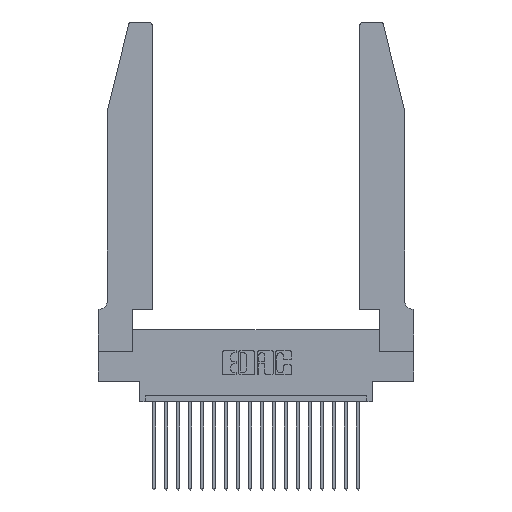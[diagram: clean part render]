
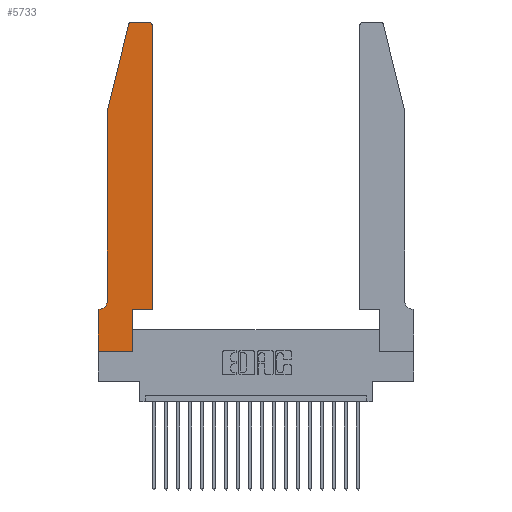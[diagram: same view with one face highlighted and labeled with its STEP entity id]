
A CAD part, top view. The second image highlights one B-rep face of the part: STEP entity #5733.
In plain terms, the highlighted planar face has unit normal (0, 0, 1).
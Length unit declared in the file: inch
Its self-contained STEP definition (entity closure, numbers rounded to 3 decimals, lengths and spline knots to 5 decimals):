
#172 = EDGE_CURVE ( 'NONE', #2098, #2395, #539, .T. ) ;
#305 = LINE ( 'NONE', #10975, #13659 ) ;
#336 = DIRECTION ( 'NONE',  ( -1., 0., 0. ) ) ;
#539 = LINE ( 'NONE', #12052, #19403 ) ;
#838 = LINE ( 'NONE', #2893, #16295 ) ;
#889 = EDGE_CURVE ( 'NONE', #14519, #3531, #14907, .T. ) ;
#1054 = EDGE_CURVE ( 'NONE', #8206, #13975, #4939, .T. ) ;
#1681 = ORIENTED_EDGE ( 'NONE', *, *, #889, .T. ) ;
#2098 = VERTEX_POINT ( 'NONE', #4313 ) ;
#2245 = ORIENTED_EDGE ( 'NONE', *, *, #15053, .T. ) ;
#2393 = AXIS2_PLACEMENT_3D ( 'NONE', #4122, #5932, #5784 ) ;
#2395 = VERTEX_POINT ( 'NONE', #18544 ) ;
#2477 = LINE ( 'NONE', #9210, #20814 ) ;
#2893 = CARTESIAN_POINT ( 'NONE',  ( 0.0755, 2., 0.37 ) ) ;
#3231 = VECTOR ( 'NONE', #336, 39.37008 ) ;
#3531 = VERTEX_POINT ( 'NONE', #12895 ) ;
#3886 = ORIENTED_EDGE ( 'NONE', *, *, #16899, .T. ) ;
#4122 = CARTESIAN_POINT ( 'NONE',  ( 0.284, 2.72, 0.37 ) ) ;
#4313 = CARTESIAN_POINT ( 'NONE',  ( 0.25487, 2.72718, 0.37 ) ) ;
#4395 = CARTESIAN_POINT ( 'NONE',  ( 0.4505, 2.72, 0.37 ) ) ;
#4397 = VERTEX_POINT ( 'NONE', #13627 ) ;
#4534 = VERTEX_POINT ( 'NONE', #5603 ) ;
#4939 = CIRCLE ( 'NONE', #19001, 0.03 ) ;
#5300 = VERTEX_POINT ( 'NONE', #20355 ) ;
#5555 = CARTESIAN_POINT ( 'NONE',  ( 0.2865, 0.35, 0.37 ) ) ;
#5599 = CARTESIAN_POINT ( 'NONE',  ( 0.0755, 0.42, 0.37 ) ) ;
#5603 = CARTESIAN_POINT ( 'NONE',  ( 0.284, 2.75, 0.37 ) ) ;
#5733 = ADVANCED_FACE ( 'NONE', ( #6633 ), #6424, .T. ) ;
#5784 = DIRECTION ( 'NONE',  ( 1., 0., 0. ) ) ;
#5795 = LINE ( 'NONE', #18187, #7918 ) ;
#5851 = DIRECTION ( 'NONE',  ( 0., -1., 0. ) ) ;
#5932 = DIRECTION ( 'NONE',  ( 0., 0., 1. ) ) ;
#6424 = PLANE ( 'NONE',  #11538 ) ;
#6446 = EDGE_CURVE ( 'NONE', #4534, #2098, #18891, .T. ) ;
#6633 = FACE_OUTER_BOUND ( 'NONE', #14360, .T. ) ;
#6716 = ORIENTED_EDGE ( 'NONE', *, *, #18861, .T. ) ;
#6823 = ORIENTED_EDGE ( 'NONE', *, *, #17131, .T. ) ;
#6986 = CARTESIAN_POINT ( 'NONE',  ( 0.2865, 0., 0.37 ) ) ;
#7301 = DIRECTION ( 'NONE',  ( 1., 0., 0. ) ) ;
#7401 = DIRECTION ( 'NONE',  ( 0., 1., 0. ) ) ;
#7745 = CARTESIAN_POINT ( 'NONE',  ( 0.4205, 2.72, 0.37 ) ) ;
#7890 = LINE ( 'NONE', #10027, #20194 ) ;
#7918 = VECTOR ( 'NONE', #15390, 39.37008 ) ;
#8206 = VERTEX_POINT ( 'NONE', #4395 ) ;
#8429 = ORIENTED_EDGE ( 'NONE', *, *, #172, .T. ) ;
#8949 = ORIENTED_EDGE ( 'NONE', *, *, #6446, .T. ) ;
#9210 = CARTESIAN_POINT ( 'NONE',  ( 0.4505, 0.35, 0.37 ) ) ;
#9518 = VECTOR ( 'NONE', #5851, 39.37008 ) ;
#10027 = CARTESIAN_POINT ( 'NONE',  ( 0.4505, 0.35, 0.37 ) ) ;
#10911 = ORIENTED_EDGE ( 'NONE', *, *, #18308, .T. ) ;
#10975 = CARTESIAN_POINT ( 'NONE',  ( 0.2605, 2.75, 0.37 ) ) ;
#11218 = CARTESIAN_POINT ( 'NONE',  ( 0.0755, 0.35, 0.37 ) ) ;
#11276 = VECTOR ( 'NONE', #7401, 39.37008 ) ;
#11538 = AXIS2_PLACEMENT_3D ( 'NONE', #20897, #17327, #7301 ) ;
#11711 = DIRECTION ( 'NONE',  ( 0., 1., 0. ) ) ;
#11729 = ORIENTED_EDGE ( 'NONE', *, *, #1054, .T. ) ;
#11818 = CIRCLE ( 'NONE', #21430, 0.07 ) ;
#11837 = DIRECTION ( 'NONE',  ( -0.239, -0.971, 0. ) ) ;
#11921 = ORIENTED_EDGE ( 'NONE', *, *, #17192, .T. ) ;
#12052 = CARTESIAN_POINT ( 'NONE',  ( 0.0755, 2., 0.37 ) ) ;
#12649 = DIRECTION ( 'NONE',  ( 1., 0., 0. ) ) ;
#12825 = CARTESIAN_POINT ( 'NONE',  ( 0., 0., 0.37 ) ) ;
#12895 = CARTESIAN_POINT ( 'NONE',  ( 0.2865, 0.35, 0.37 ) ) ;
#13002 = CARTESIAN_POINT ( 'NONE',  ( 0., 0., 0.37 ) ) ;
#13627 = CARTESIAN_POINT ( 'NONE',  ( 0., 0.35, 0.37 ) ) ;
#13659 = VECTOR ( 'NONE', #17476, 39.37008 ) ;
#13729 = ORIENTED_EDGE ( 'NONE', *, *, #19176, .T. ) ;
#13965 = LINE ( 'NONE', #11218, #3231 ) ;
#13975 = VERTEX_POINT ( 'NONE', #14861 ) ;
#14001 = DIRECTION ( 'NONE',  ( 0., 0., -1. ) ) ;
#14174 = CARTESIAN_POINT ( 'NONE',  ( 0.0055, 0.35, 0.37 ) ) ;
#14360 = EDGE_LOOP ( 'NONE', ( #3886, #8949, #8429, #6823, #17408, #10911, #13729, #6716, #1681, #2245, #11921, #11729 ) ) ;
#14519 = VERTEX_POINT ( 'NONE', #6986 ) ;
#14688 = DIRECTION ( 'NONE',  ( 0., 0., 1. ) ) ;
#14861 = CARTESIAN_POINT ( 'NONE',  ( 0.4205, 2.75, 0.37 ) ) ;
#14907 = LINE ( 'NONE', #5555, #11276 ) ;
#15002 = VERTEX_POINT ( 'NONE', #14174 ) ;
#15053 = EDGE_CURVE ( 'NONE', #3531, #5300, #2477, .T. ) ;
#15390 = DIRECTION ( 'NONE',  ( 1., 0., 0. ) ) ;
#15679 = DIRECTION ( 'NONE',  ( -1., 0., 0. ) ) ;
#15904 = VERTEX_POINT ( 'NONE', #5599 ) ;
#16295 = VECTOR ( 'NONE', #21054, 39.37008 ) ;
#16899 = EDGE_CURVE ( 'NONE', #13975, #4534, #305, .T. ) ;
#17131 = EDGE_CURVE ( 'NONE', #2395, #15904, #838, .T. ) ;
#17192 = EDGE_CURVE ( 'NONE', #5300, #8206, #7890, .T. ) ;
#17327 = DIRECTION ( 'NONE',  ( 0., 0., 1. ) ) ;
#17408 = ORIENTED_EDGE ( 'NONE', *, *, #20351, .T. ) ;
#17476 = DIRECTION ( 'NONE',  ( -1., 0., 0. ) ) ;
#18187 = CARTESIAN_POINT ( 'NONE',  ( 0., 0., 0.37 ) ) ;
#18308 = EDGE_CURVE ( 'NONE', #15002, #4397, #13965, .T. ) ;
#18544 = CARTESIAN_POINT ( 'NONE',  ( 0.0755, 2., 0.37 ) ) ;
#18861 = EDGE_CURVE ( 'NONE', #21311, #14519, #5795, .T. ) ;
#18881 = CARTESIAN_POINT ( 'NONE',  ( 0.0055, 0.42, 0.37 ) ) ;
#18891 = CIRCLE ( 'NONE', #2393, 0.03 ) ;
#19001 = AXIS2_PLACEMENT_3D ( 'NONE', #7745, #14688, #21115 ) ;
#19176 = EDGE_CURVE ( 'NONE', #4397, #21311, #21232, .T. ) ;
#19403 = VECTOR ( 'NONE', #11837, 39.37008 ) ;
#20194 = VECTOR ( 'NONE', #11711, 39.37008 ) ;
#20351 = EDGE_CURVE ( 'NONE', #15904, #15002, #11818, .T. ) ;
#20355 = CARTESIAN_POINT ( 'NONE',  ( 0.4505, 0.35, 0.37 ) ) ;
#20814 = VECTOR ( 'NONE', #12649, 39.37008 ) ;
#20897 = CARTESIAN_POINT ( 'NONE',  ( 0., 0.35, 0.37 ) ) ;
#21054 = DIRECTION ( 'NONE',  ( 0., -1., 0. ) ) ;
#21115 = DIRECTION ( 'NONE',  ( 1., 0., 0. ) ) ;
#21232 = LINE ( 'NONE', #12825, #9518 ) ;
#21311 = VERTEX_POINT ( 'NONE', #13002 ) ;
#21430 = AXIS2_PLACEMENT_3D ( 'NONE', #18881, #14001, #15679 ) ;
